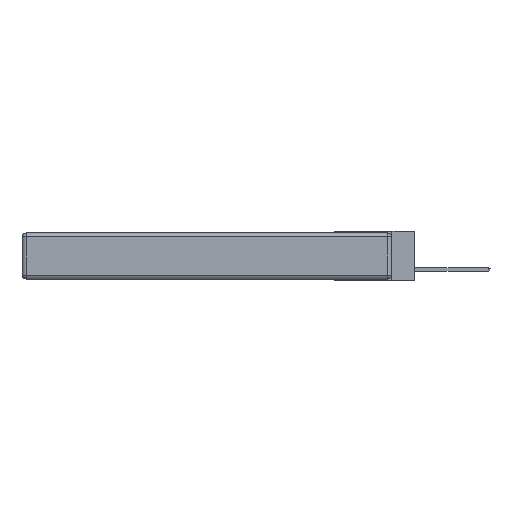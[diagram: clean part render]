
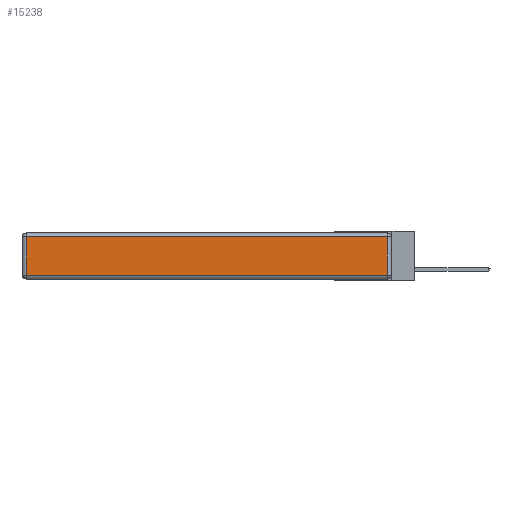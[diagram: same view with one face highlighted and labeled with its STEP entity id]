
A CAD part, left-side view. The second image highlights one B-rep face of the part: STEP entity #15238.
In plain terms, the highlighted planar face has unit normal (-1, 0, 0).
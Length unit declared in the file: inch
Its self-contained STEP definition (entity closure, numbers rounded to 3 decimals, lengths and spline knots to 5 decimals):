
#637 = VERTEX_POINT ( 'NONE', #17264 ) ;
#886 = LINE ( 'NONE', #4742, #14428 ) ;
#1558 = DIRECTION ( 'NONE',  ( 0., 0., 1. ) ) ;
#3974 = ORIENTED_EDGE ( 'NONE', *, *, #17092, .T. ) ;
#4742 = CARTESIAN_POINT ( 'NONE',  ( 0., 2.72, -0.343 ) ) ;
#4972 = CARTESIAN_POINT ( 'NONE',  ( 0., 0.03, -0.313 ) ) ;
#5246 = VERTEX_POINT ( 'NONE', #5351 ) ;
#5351 = CARTESIAN_POINT ( 'NONE',  ( 0., 2.72, -0.03 ) ) ;
#6443 = DIRECTION ( 'NONE',  ( 0., 0., 1. ) ) ;
#6531 = LINE ( 'NONE', #10022, #12197 ) ;
#6813 = VECTOR ( 'NONE', #1558, 39.37008 ) ;
#7020 = DIRECTION ( 'NONE',  ( 0., 0., -1. ) ) ;
#7496 = VERTEX_POINT ( 'NONE', #4972 ) ;
#9166 = EDGE_CURVE ( 'NONE', #7496, #14964, #9639, .T. ) ;
#9352 = EDGE_CURVE ( 'NONE', #14964, #5246, #6531, .T. ) ;
#9534 = ORIENTED_EDGE ( 'NONE', *, *, #9352, .T. ) ;
#9639 = LINE ( 'NONE', #21208, #6813 ) ;
#10022 = CARTESIAN_POINT ( 'NONE',  ( 0., 2.75, -0.03 ) ) ;
#10517 = LINE ( 'NONE', #18464, #14053 ) ;
#11869 = FACE_OUTER_BOUND ( 'NONE', #15955, .T. ) ;
#12197 = VECTOR ( 'NONE', #18417, 39.37008 ) ;
#12995 = CARTESIAN_POINT ( 'NONE',  ( 0., 0.03, -0.03 ) ) ;
#13943 = EDGE_CURVE ( 'NONE', #5246, #637, #886, .T. ) ;
#14053 = VECTOR ( 'NONE', #16896, 39.37008 ) ;
#14428 = VECTOR ( 'NONE', #7020, 39.37008 ) ;
#14541 = CARTESIAN_POINT ( 'NONE',  ( 0., 0., -0.343 ) ) ;
#14964 = VERTEX_POINT ( 'NONE', #12995 ) ;
#15238 = ADVANCED_FACE ( 'NONE', ( #11869 ), #16284, .T. ) ;
#15955 = EDGE_LOOP ( 'NONE', ( #3974, #17859, #9534, #19581 ) ) ;
#16284 = PLANE ( 'NONE',  #19503 ) ;
#16896 = DIRECTION ( 'NONE',  ( 0., -1., 0. ) ) ;
#17092 = EDGE_CURVE ( 'NONE', #637, #7496, #10517, .T. ) ;
#17264 = CARTESIAN_POINT ( 'NONE',  ( 0., 2.72, -0.313 ) ) ;
#17859 = ORIENTED_EDGE ( 'NONE', *, *, #9166, .T. ) ;
#18417 = DIRECTION ( 'NONE',  ( 0., 1., 0. ) ) ;
#18464 = CARTESIAN_POINT ( 'NONE',  ( 0., 0., -0.313 ) ) ;
#19457 = DIRECTION ( 'NONE',  ( -1., 0., 0. ) ) ;
#19503 = AXIS2_PLACEMENT_3D ( 'NONE', #14541, #19457, #6443 ) ;
#19581 = ORIENTED_EDGE ( 'NONE', *, *, #13943, .T. ) ;
#21208 = CARTESIAN_POINT ( 'NONE',  ( 0., 0.03, -0.343 ) ) ;
